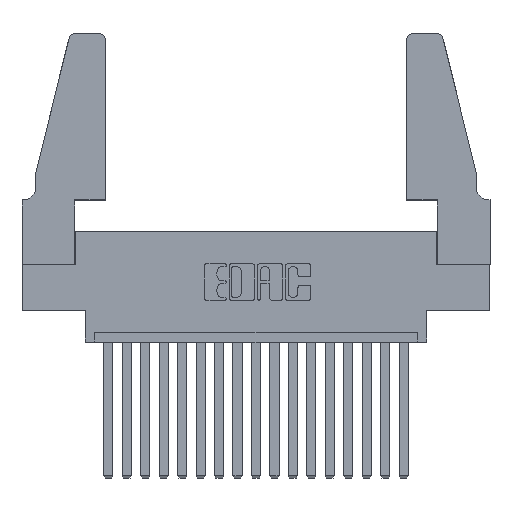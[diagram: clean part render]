
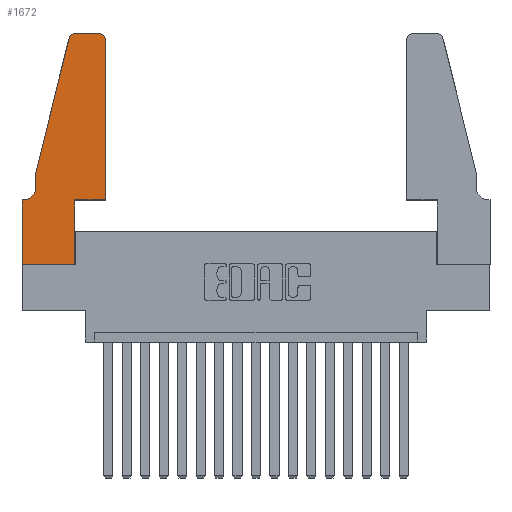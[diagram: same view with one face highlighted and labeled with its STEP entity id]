
A CAD part, top view. The second image highlights one B-rep face of the part: STEP entity #1672.
In plain terms, the highlighted planar face has unit normal (0, 0, 1).
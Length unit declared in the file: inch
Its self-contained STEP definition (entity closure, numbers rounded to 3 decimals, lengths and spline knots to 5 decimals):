
#231 = CARTESIAN_POINT ( 'NONE',  ( 0.0755, 0.5, 0.37 ) ) ;
#250 = CARTESIAN_POINT ( 'NONE',  ( 0.0755, 0.35, 0.37 ) ) ;
#918 = ORIENTED_EDGE ( 'NONE', *, *, #5124, .T. ) ;
#1153 = ORIENTED_EDGE ( 'NONE', *, *, #4387, .T. ) ;
#1418 = DIRECTION ( 'NONE',  ( -1., 0., 0. ) ) ;
#1579 = CIRCLE ( 'NONE', #15245, 0.07 ) ;
#1645 = DIRECTION ( 'NONE',  ( 0., -1., 0. ) ) ;
#1672 = ADVANCED_FACE ( 'NONE', ( #17600 ), #4500, .T. ) ;
#1930 = VECTOR ( 'NONE', #14512, 39.37008 ) ;
#2146 = CARTESIAN_POINT ( 'NONE',  ( 0.0755, 0.42, 0.37 ) ) ;
#2313 = LINE ( 'NONE', #18074, #5869 ) ;
#2355 = EDGE_CURVE ( 'NONE', #13866, #6744, #14700, .T. ) ;
#2857 = DIRECTION ( 'NONE',  ( 0., 0., 1. ) ) ;
#3018 = VERTEX_POINT ( 'NONE', #15596 ) ;
#3320 = VERTEX_POINT ( 'NONE', #10442 ) ;
#3456 = LINE ( 'NONE', #4617, #1930 ) ;
#3503 = ORIENTED_EDGE ( 'NONE', *, *, #16092, .T. ) ;
#3553 = EDGE_CURVE ( 'NONE', #3018, #7730, #9374, .T. ) ;
#3815 = CIRCLE ( 'NONE', #8679, 0.03 ) ;
#3941 = DIRECTION ( 'NONE',  ( 1., 0., 0. ) ) ;
#4033 = AXIS2_PLACEMENT_3D ( 'NONE', #14271, #15825, #11486 ) ;
#4344 = VERTEX_POINT ( 'NONE', #5856 ) ;
#4387 = EDGE_CURVE ( 'NONE', #6888, #4981, #15799, .T. ) ;
#4500 = PLANE ( 'NONE',  #4033 ) ;
#4617 = CARTESIAN_POINT ( 'NONE',  ( 0.4505, 0.35, 0.37 ) ) ;
#4950 = CARTESIAN_POINT ( 'NONE',  ( 0.0055, 0.35, 0.37 ) ) ;
#4981 = VERTEX_POINT ( 'NONE', #6977 ) ;
#4989 = EDGE_CURVE ( 'NONE', #6744, #4344, #12437, .T. ) ;
#5124 = EDGE_CURVE ( 'NONE', #5744, #13866, #3815, .T. ) ;
#5253 = DIRECTION ( 'NONE',  ( 0., 1., 0. ) ) ;
#5714 = CARTESIAN_POINT ( 'NONE',  ( 0.2865, 0., 0.37 ) ) ;
#5744 = VERTEX_POINT ( 'NONE', #17431 ) ;
#5856 = CARTESIAN_POINT ( 'NONE',  ( 0.25487, 1.22718, 0.37 ) ) ;
#5869 = VECTOR ( 'NONE', #9603, 39.37008 ) ;
#6382 = VECTOR ( 'NONE', #5253, 39.37008 ) ;
#6420 = EDGE_CURVE ( 'NONE', #4981, #3018, #7708, .T. ) ;
#6438 = CARTESIAN_POINT ( 'NONE',  ( 0.4505, 0.35, 0.37 ) ) ;
#6446 = ORIENTED_EDGE ( 'NONE', *, *, #4989, .T. ) ;
#6513 = VECTOR ( 'NONE', #3941, 39.37008 ) ;
#6744 = VERTEX_POINT ( 'NONE', #13141 ) ;
#6888 = VERTEX_POINT ( 'NONE', #4950 ) ;
#6977 = CARTESIAN_POINT ( 'NONE',  ( 0., 0.35, 0.37 ) ) ;
#7255 = LINE ( 'NONE', #6438, #6382 ) ;
#7267 = ORIENTED_EDGE ( 'NONE', *, *, #17984, .T. ) ;
#7268 = VECTOR ( 'NONE', #12573, 39.37008 ) ;
#7279 = ORIENTED_EDGE ( 'NONE', *, *, #3553, .T. ) ;
#7394 = ORIENTED_EDGE ( 'NONE', *, *, #13451, .T. ) ;
#7457 = ORIENTED_EDGE ( 'NONE', *, *, #16577, .T. ) ;
#7473 = CARTESIAN_POINT ( 'NONE',  ( 0.4205, 1.22, 0.37 ) ) ;
#7708 = LINE ( 'NONE', #12512, #7268 ) ;
#7730 = VERTEX_POINT ( 'NONE', #5714 ) ;
#8066 = ORIENTED_EDGE ( 'NONE', *, *, #6420, .T. ) ;
#8413 = CARTESIAN_POINT ( 'NONE',  ( 0.2865, 0.35, 0.37 ) ) ;
#8679 = AXIS2_PLACEMENT_3D ( 'NONE', #7473, #10075, #8829 ) ;
#8829 = DIRECTION ( 'NONE',  ( 1., 0., 0. ) ) ;
#9374 = LINE ( 'NONE', #17859, #6513 ) ;
#9603 = DIRECTION ( 'NONE',  ( -0.239, -0.971, 0. ) ) ;
#9646 = VERTEX_POINT ( 'NONE', #8413 ) ;
#9954 = DIRECTION ( 'NONE',  ( 1., 0., 0. ) ) ;
#10075 = DIRECTION ( 'NONE',  ( 0., 0., 1. ) ) ;
#10121 = DIRECTION ( 'NONE',  ( -1., 0., 0. ) ) ;
#10357 = DIRECTION ( 'NONE',  ( 0., 1., 0. ) ) ;
#10442 = CARTESIAN_POINT ( 'NONE',  ( 0.4505, 0.35, 0.37 ) ) ;
#10724 = VECTOR ( 'NONE', #10357, 39.37008 ) ;
#11153 = VERTEX_POINT ( 'NONE', #17180 ) ;
#11324 = CARTESIAN_POINT ( 'NONE',  ( 0.284, 1.22, 0.37 ) ) ;
#11486 = DIRECTION ( 'NONE',  ( 1., 0., 0. ) ) ;
#11910 = CARTESIAN_POINT ( 'NONE',  ( 0.2865, 0.35, 0.37 ) ) ;
#11921 = VECTOR ( 'NONE', #1645, 39.37008 ) ;
#12437 = CIRCLE ( 'NONE', #16287, 0.03 ) ;
#12512 = CARTESIAN_POINT ( 'NONE',  ( 0., 0., 0.37 ) ) ;
#12573 = DIRECTION ( 'NONE',  ( 0., -1., 0. ) ) ;
#13141 = CARTESIAN_POINT ( 'NONE',  ( 0.284, 1.25, 0.37 ) ) ;
#13163 = EDGE_CURVE ( 'NONE', #7730, #9646, #14945, .T. ) ;
#13275 = CARTESIAN_POINT ( 'NONE',  ( 0.4205, 1.25, 0.37 ) ) ;
#13276 = VERTEX_POINT ( 'NONE', #2146 ) ;
#13451 = EDGE_CURVE ( 'NONE', #4344, #11153, #2313, .T. ) ;
#13866 = VERTEX_POINT ( 'NONE', #13275 ) ;
#14271 = CARTESIAN_POINT ( 'NONE',  ( 0., 0.35, 0.37 ) ) ;
#14347 = CARTESIAN_POINT ( 'NONE',  ( 0.0055, 0.42, 0.37 ) ) ;
#14512 = DIRECTION ( 'NONE',  ( 1., 0., 0. ) ) ;
#14700 = LINE ( 'NONE', #16906, #15376 ) ;
#14945 = LINE ( 'NONE', #11910, #10724 ) ;
#14952 = EDGE_LOOP ( 'NONE', ( #15841, #6446, #7394, #7457, #3503, #1153, #8066, #7279, #16139, #7267, #16604, #918 ) ) ;
#15245 = AXIS2_PLACEMENT_3D ( 'NONE', #14347, #15778, #10121 ) ;
#15351 = VECTOR ( 'NONE', #15752, 39.37008 ) ;
#15376 = VECTOR ( 'NONE', #1418, 39.37008 ) ;
#15477 = LINE ( 'NONE', #231, #11921 ) ;
#15596 = CARTESIAN_POINT ( 'NONE',  ( 0., 0., 0.37 ) ) ;
#15752 = DIRECTION ( 'NONE',  ( -1., 0., 0. ) ) ;
#15778 = DIRECTION ( 'NONE',  ( 0., 0., -1. ) ) ;
#15799 = LINE ( 'NONE', #250, #15351 ) ;
#15825 = DIRECTION ( 'NONE',  ( 0., 0., 1. ) ) ;
#15841 = ORIENTED_EDGE ( 'NONE', *, *, #2355, .T. ) ;
#16092 = EDGE_CURVE ( 'NONE', #13276, #6888, #1579, .T. ) ;
#16139 = ORIENTED_EDGE ( 'NONE', *, *, #13163, .T. ) ;
#16287 = AXIS2_PLACEMENT_3D ( 'NONE', #11324, #2857, #9954 ) ;
#16577 = EDGE_CURVE ( 'NONE', #11153, #13276, #15477, .T. ) ;
#16604 = ORIENTED_EDGE ( 'NONE', *, *, #16894, .T. ) ;
#16894 = EDGE_CURVE ( 'NONE', #3320, #5744, #7255, .T. ) ;
#16906 = CARTESIAN_POINT ( 'NONE',  ( 0.2605, 1.25, 0.37 ) ) ;
#17180 = CARTESIAN_POINT ( 'NONE',  ( 0.0755, 0.5, 0.37 ) ) ;
#17431 = CARTESIAN_POINT ( 'NONE',  ( 0.4505, 1.22, 0.37 ) ) ;
#17600 = FACE_OUTER_BOUND ( 'NONE', #14952, .T. ) ;
#17859 = CARTESIAN_POINT ( 'NONE',  ( 0., 0., 0.37 ) ) ;
#17984 = EDGE_CURVE ( 'NONE', #9646, #3320, #3456, .T. ) ;
#18074 = CARTESIAN_POINT ( 'NONE',  ( 0.0755, 0.5, 0.37 ) ) ;
